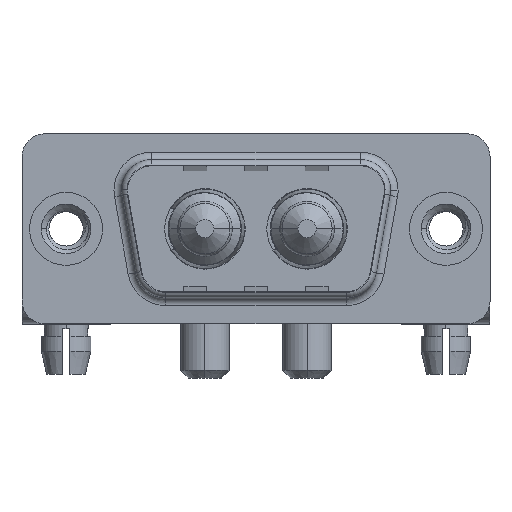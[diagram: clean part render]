
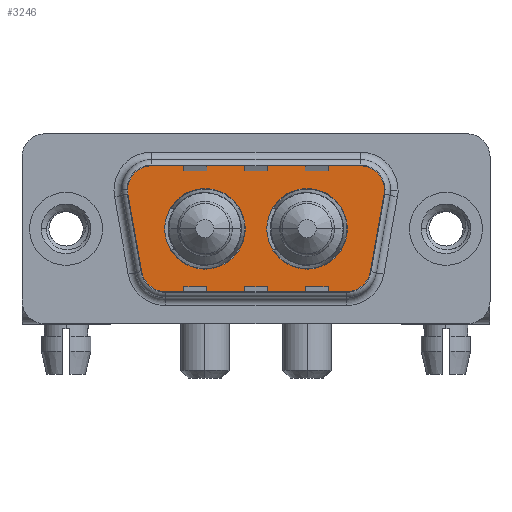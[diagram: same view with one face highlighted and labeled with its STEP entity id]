
A CAD part, top view. The second image highlights one B-rep face of the part: STEP entity #3246.
In plain terms, the highlighted planar face has unit normal (0, 0, 1).
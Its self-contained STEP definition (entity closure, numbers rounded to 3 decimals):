
#49 = DIRECTION ( 'NONE',  ( 1., 0., 0. ) ) ;
#99 = CIRCLE ( 'NONE', #3304, 2.65 ) ;
#105 = DIRECTION ( 'NONE',  ( 0., 0., 1. ) ) ;
#203 = DIRECTION ( 'NONE',  ( -1., 0., 0. ) ) ;
#228 = DIRECTION ( 'NONE',  ( 1., 0., 0. ) ) ;
#383 = EDGE_LOOP ( 'NONE', ( #1695, #3481, #13517, #9724, #4082, #9913, #4535, #2024, #5206 ) ) ;
#426 = EDGE_CURVE ( 'NONE', #13658, #5623, #12107, .T. ) ;
#607 = CARTESIAN_POINT ( 'NONE',  ( 11.79, 0., 0. ) ) ;
#770 = DIRECTION ( 'NONE',  ( 0., 0., 1. ) ) ;
#815 = DIRECTION ( 'NONE',  ( 1., 0., 0. ) ) ;
#844 = EDGE_CURVE ( 'NONE', #4879, #7107, #1761, .T. ) ;
#873 = VERTEX_POINT ( 'NONE', #2979 ) ;
#902 = CARTESIAN_POINT ( 'NONE',  ( 21.534, 2.553, 0. ) ) ;
#985 = DIRECTION ( 'NONE',  ( 0., 0., 1. ) ) ;
#1133 = CARTESIAN_POINT ( 'NONE',  ( 18.541, -2.9, 0. ) ) ;
#1153 = CARTESIAN_POINT ( 'NONE',  ( 21.534, 2.553, 0. ) ) ;
#1392 = CARTESIAN_POINT ( 'NONE',  ( 18.541, -2.9, 0. ) ) ;
#1609 = AXIS2_PLACEMENT_3D ( 'NONE', #5434, #3169, #7371 ) ;
#1626 = DIRECTION ( 'NONE',  ( 1., 0., 0. ) ) ;
#1692 = EDGE_CURVE ( 'NONE', #6145, #873, #6054, .T. ) ;
#1695 = ORIENTED_EDGE ( 'NONE', *, *, #5043, .T. ) ;
#1714 = AXIS2_PLACEMENT_3D ( 'NONE', #11908, #10918, #49 ) ;
#1716 = CARTESIAN_POINT ( 'NONE',  ( 20.511, -3.247, 0. ) ) ;
#1761 = CIRCLE ( 'NONE', #5843, 2. ) ;
#1773 = CARTESIAN_POINT ( 'NONE',  ( 6.459, -4.9, 0. ) ) ;
#1979 = AXIS2_PLACEMENT_3D ( 'NONE', #1133, #105, #11120 ) ;
#2024 = ORIENTED_EDGE ( 'NONE', *, *, #844, .T. ) ;
#2033 = DIRECTION ( 'NONE',  ( -1., 0., 0. ) ) ;
#2068 = CARTESIAN_POINT ( 'NONE',  ( 5.436, 2.9, 0. ) ) ;
#2078 = CARTESIAN_POINT ( 'NONE',  ( 3.466, 2.553, 0. ) ) ;
#2353 = VECTOR ( 'NONE', #1626, 1000. ) ;
#2671 = CIRCLE ( 'NONE', #1979, 2. ) ;
#2957 = EDGE_CURVE ( 'NONE', #873, #6145, #6368, .T. ) ;
#2979 = CARTESIAN_POINT ( 'NONE',  ( 13.21, 0., 0. ) ) ;
#3074 = CARTESIAN_POINT ( 'NONE',  ( 9.14, 0., 0. ) ) ;
#3169 = DIRECTION ( 'NONE',  ( 0., 0., 1. ) ) ;
#3213 = LINE ( 'NONE', #6626, #9678 ) ;
#3246 = ADVANCED_FACE ( 'NONE', ( #8807, #5722, #11168 ), #13155, .T. ) ;
#3304 = AXIS2_PLACEMENT_3D ( 'NONE', #3074, #5270, #13863 ) ;
#3377 = DIRECTION ( 'NONE',  ( 0., 0., 1. ) ) ;
#3481 = ORIENTED_EDGE ( 'NONE', *, *, #4170, .T. ) ;
#3540 = CARTESIAN_POINT ( 'NONE',  ( 9.14, 0., 0. ) ) ;
#3541 = AXIS2_PLACEMENT_3D ( 'NONE', #1392, #3377, #228 ) ;
#3920 = DIRECTION ( 'NONE',  ( -1., 0., 0. ) ) ;
#3933 = VECTOR ( 'NONE', #9770, 1000. ) ;
#4053 = DIRECTION ( 'NONE',  ( 0., 0., 1. ) ) ;
#4082 = ORIENTED_EDGE ( 'NONE', *, *, #11138, .T. ) ;
#4170 = EDGE_CURVE ( 'NONE', #6645, #12957, #6378, .T. ) ;
#4535 = ORIENTED_EDGE ( 'NONE', *, *, #6509, .T. ) ;
#4754 = AXIS2_PLACEMENT_3D ( 'NONE', #9479, #4053, #3920 ) ;
#4871 = VERTEX_POINT ( 'NONE', #4923 ) ;
#4879 = VERTEX_POINT ( 'NONE', #13643 ) ;
#4903 = CARTESIAN_POINT ( 'NONE',  ( 5.436, 4.9, 0. ) ) ;
#4923 = CARTESIAN_POINT ( 'NONE',  ( 18.541, -4.9, 0. ) ) ;
#5043 = EDGE_CURVE ( 'NONE', #4871, #6645, #2671, .T. ) ;
#5206 = ORIENTED_EDGE ( 'NONE', *, *, #7227, .T. ) ;
#5270 = DIRECTION ( 'NONE',  ( 0., 0., 1. ) ) ;
#5357 = DIRECTION ( 'NONE',  ( 0., 0., 1. ) ) ;
#5434 = CARTESIAN_POINT ( 'NONE',  ( 15.86, 0., 0. ) ) ;
#5623 = VERTEX_POINT ( 'NONE', #10651 ) ;
#5722 = FACE_BOUND ( 'NONE', #7217, .T. ) ;
#5782 = CARTESIAN_POINT ( 'NONE',  ( 19.564, 4.9, 0. ) ) ;
#5812 = EDGE_LOOP ( 'NONE', ( #13908, #13021 ) ) ;
#5843 = AXIS2_PLACEMENT_3D ( 'NONE', #12684, #770, #12472 ) ;
#5947 = AXIS2_PLACEMENT_3D ( 'NONE', #2068, #985, #6262 ) ;
#5955 = VERTEX_POINT ( 'NONE', #607 ) ;
#6044 = AXIS2_PLACEMENT_3D ( 'NONE', #6366, #12138, #2033 ) ;
#6054 = CIRCLE ( 'NONE', #1714, 2.65 ) ;
#6145 = VERTEX_POINT ( 'NONE', #6423 ) ;
#6262 = DIRECTION ( 'NONE',  ( 1., 0., 0. ) ) ;
#6301 = VERTEX_POINT ( 'NONE', #6997 ) ;
#6366 = CARTESIAN_POINT ( 'NONE',  ( 19.564, 2.9, 0. ) ) ;
#6368 = CIRCLE ( 'NONE', #1609, 2.65 ) ;
#6378 = LINE ( 'NONE', #902, #10386 ) ;
#6423 = CARTESIAN_POINT ( 'NONE',  ( 18.51, 0., 0. ) ) ;
#6509 = EDGE_CURVE ( 'NONE', #5623, #4879, #11845, .T. ) ;
#6542 = ORIENTED_EDGE ( 'NONE', *, *, #10343, .F. ) ;
#6626 = CARTESIAN_POINT ( 'NONE',  ( 5.436, 4.9, 0. ) ) ;
#6645 = VERTEX_POINT ( 'NONE', #1716 ) ;
#6959 = CIRCLE ( 'NONE', #6044, 2. ) ;
#6997 = CARTESIAN_POINT ( 'NONE',  ( 6.49, 0., 0. ) ) ;
#7107 = VERTEX_POINT ( 'NONE', #12463 ) ;
#7217 = EDGE_LOOP ( 'NONE', ( #7742, #6542 ) ) ;
#7227 = EDGE_CURVE ( 'NONE', #7107, #4871, #9393, .T. ) ;
#7371 = DIRECTION ( 'NONE',  ( 1., 0., 0. ) ) ;
#7705 = CIRCLE ( 'NONE', #4754, 2. ) ;
#7742 = ORIENTED_EDGE ( 'NONE', *, *, #10946, .F. ) ;
#8534 = AXIS2_PLACEMENT_3D ( 'NONE', #3540, #5357, #815 ) ;
#8807 = FACE_BOUND ( 'NONE', #5812, .T. ) ;
#9393 = LINE ( 'NONE', #1773, #2353 ) ;
#9479 = CARTESIAN_POINT ( 'NONE',  ( 19.564, 2.9, 0. ) ) ;
#9678 = VECTOR ( 'NONE', #203, 1000. ) ;
#9724 = ORIENTED_EDGE ( 'NONE', *, *, #11515, .T. ) ;
#9770 = DIRECTION ( 'NONE',  ( 0.174, -0.985, 0. ) ) ;
#9913 = ORIENTED_EDGE ( 'NONE', *, *, #426, .T. ) ;
#10017 = EDGE_CURVE ( 'NONE', #12957, #12340, #7705, .T. ) ;
#10272 = CARTESIAN_POINT ( 'NONE',  ( 21.564, 2.9, 0. ) ) ;
#10343 = EDGE_CURVE ( 'NONE', #6301, #5955, #11283, .T. ) ;
#10386 = VECTOR ( 'NONE', #13827, 1000. ) ;
#10651 = CARTESIAN_POINT ( 'NONE',  ( 3.466, 2.553, 0. ) ) ;
#10826 = VERTEX_POINT ( 'NONE', #5782 ) ;
#10918 = DIRECTION ( 'NONE',  ( 0., 0., 1. ) ) ;
#10946 = EDGE_CURVE ( 'NONE', #5955, #6301, #99, .T. ) ;
#11120 = DIRECTION ( 'NONE',  ( 1., 0., 0. ) ) ;
#11138 = EDGE_CURVE ( 'NONE', #10826, #13658, #3213, .T. ) ;
#11168 = FACE_OUTER_BOUND ( 'NONE', #383, .T. ) ;
#11283 = CIRCLE ( 'NONE', #8534, 2.65 ) ;
#11515 = EDGE_CURVE ( 'NONE', #12340, #10826, #6959, .T. ) ;
#11845 = LINE ( 'NONE', #2078, #3933 ) ;
#11908 = CARTESIAN_POINT ( 'NONE',  ( 15.86, 0., 0. ) ) ;
#12107 = CIRCLE ( 'NONE', #5947, 2. ) ;
#12138 = DIRECTION ( 'NONE',  ( 0., 0., 1. ) ) ;
#12340 = VERTEX_POINT ( 'NONE', #10272 ) ;
#12463 = CARTESIAN_POINT ( 'NONE',  ( 6.459, -4.9, 0. ) ) ;
#12472 = DIRECTION ( 'NONE',  ( -1., 0., 0. ) ) ;
#12684 = CARTESIAN_POINT ( 'NONE',  ( 6.459, -2.9, 0. ) ) ;
#12957 = VERTEX_POINT ( 'NONE', #1153 ) ;
#13021 = ORIENTED_EDGE ( 'NONE', *, *, #2957, .F. ) ;
#13155 = PLANE ( 'NONE',  #3541 ) ;
#13517 = ORIENTED_EDGE ( 'NONE', *, *, #10017, .T. ) ;
#13643 = CARTESIAN_POINT ( 'NONE',  ( 4.489, -3.247, 0. ) ) ;
#13658 = VERTEX_POINT ( 'NONE', #4903 ) ;
#13827 = DIRECTION ( 'NONE',  ( 0.174, 0.985, 0. ) ) ;
#13863 = DIRECTION ( 'NONE',  ( 1., 0., 0. ) ) ;
#13908 = ORIENTED_EDGE ( 'NONE', *, *, #1692, .F. ) ;
